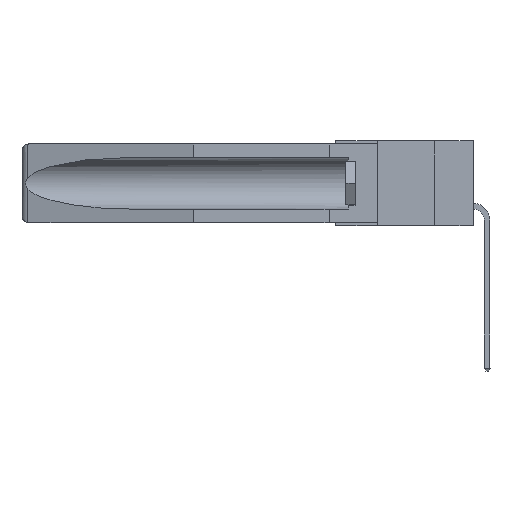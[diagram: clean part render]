
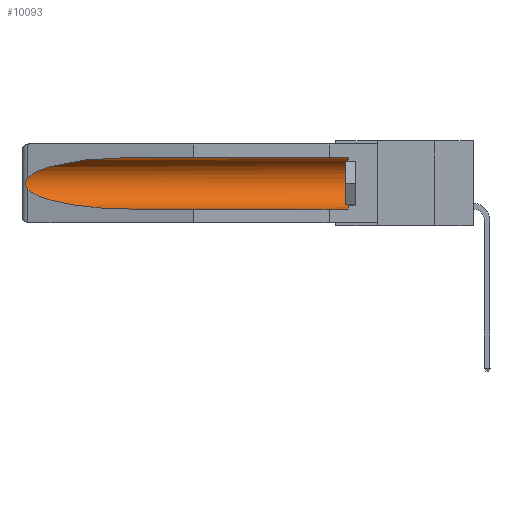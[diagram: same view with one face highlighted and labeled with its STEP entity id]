
A CAD part, left-side view. The second image highlights one B-rep face of the part: STEP entity #10093.
In plain terms, the highlighted cylindrical face has radius 2.857 mm (diameter 5.715 mm), a partial arc.
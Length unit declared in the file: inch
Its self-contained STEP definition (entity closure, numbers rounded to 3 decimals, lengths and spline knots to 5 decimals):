
#797 = VERTEX_POINT ( 'NONE', #23569 ) ;
#885 = AXIS2_PLACEMENT_3D ( 'NONE', #16481, #24147, #20278 ) ;
#1454 = CARTESIAN_POINT ( 'NONE',  ( 0.26654, 1.53092, -0.15636 ) ) ;
#1532 = CARTESIAN_POINT ( 'NONE',  ( 0.2673, 1.53269, -0.17917 ) ) ;
#1546 = DIRECTION ( 'NONE',  ( 0., 1., 0. ) ) ;
#2157 = LINE ( 'NONE', #13804, #13499 ) ;
#2451 = ORIENTED_EDGE ( 'NONE', *, *, #18978, .T. ) ;
#3432 = CARTESIAN_POINT ( 'NONE',  ( 0.2675, 1.53308, -0.17534 ) ) ;
#3751 = CARTESIAN_POINT ( 'NONE',  ( 0.155, -0.30754, -0.1715 ) ) ;
#5003 =( BOUNDED_CURVE ( )  B_SPLINE_CURVE ( 3, ( #21519, #23623, #23539, #6276 ),
 .UNSPECIFIED., .F., .F. ) 
 B_SPLINE_CURVE_WITH_KNOTS ( ( 4, 4 ),
 ( 4.71239, 6.08839 ),
 .UNSPECIFIED. ) 
 CURVE ( )  GEOMETRIC_REPRESENTATION_ITEM ( )  RATIONAL_B_SPLINE_CURVE ( ( 1., 0.848, 0.848, 1. ) ) 
 REPRESENTATION_ITEM ( '' )  );
#5184 = CARTESIAN_POINT ( 'NONE',  ( 0.26597, 1.52961, -0.15275 ) ) ;
#5522 = CARTESIAN_POINT ( 'NONE',  ( 0.155, -0.30754, -0.059 ) ) ;
#5942 = CARTESIAN_POINT ( 'NONE',  ( 0.26537, 1.52718, -0.19328 ) ) ;
#6276 = CARTESIAN_POINT ( 'NONE',  ( 0.26537, 1.52718, -0.14972 ) ) ;
#7214 = VERTEX_POINT ( 'NONE', #7728 ) ;
#7616 =( BOUNDED_CURVE ( )  B_SPLINE_CURVE ( 3, ( #5942, #23096, #16037, #16194 ),
 .UNSPECIFIED., .F., .T. ) 
 B_SPLINE_CURVE_WITH_KNOTS ( ( 4, 4 ),
 ( 0.1948, 1.5708 ),
 .UNSPECIFIED. ) 
 CURVE ( )  GEOMETRIC_REPRESENTATION_ITEM ( )  RATIONAL_B_SPLINE_CURVE ( ( 1., 0.848, 0.848, 1. ) ) 
 REPRESENTATION_ITEM ( '' )  );
#7728 = CARTESIAN_POINT ( 'NONE',  ( 0.155, 1.07973, -0.059 ) ) ;
#9134 = ORIENTED_EDGE ( 'NONE', *, *, #12036, .F. ) ;
#9260 = CARTESIAN_POINT ( 'NONE',  ( 0.155, 1.07973, -0.284 ) ) ;
#9753 = DIRECTION ( 'NONE',  ( 0., 1., 0. ) ) ;
#9761 = VERTEX_POINT ( 'NONE', #20776 ) ;
#10093 = ADVANCED_FACE ( 'NONE', ( #23788 ), #19289, .F. ) ;
#10319 = DIRECTION ( 'NONE',  ( 0., 1., 0. ) ) ;
#10331 = EDGE_LOOP ( 'NONE', ( #11541, #17048, #2451, #9134, #21448, #16360 ) ) ;
#10342 = VERTEX_POINT ( 'NONE', #13432 ) ;
#10353 = CIRCLE ( 'NONE', #885, 0.1125 ) ;
#11541 = ORIENTED_EDGE ( 'NONE', *, *, #14503, .T. ) ;
#11662 = DIRECTION ( 'NONE',  ( 0., 0., 1. ) ) ;
#12036 = EDGE_CURVE ( 'NONE', #14965, #22515, #2157, .T. ) ;
#12930 = CARTESIAN_POINT ( 'NONE',  ( 0.2675, 1.53308, -0.16763 ) ) ;
#12991 = AXIS2_PLACEMENT_3D ( 'NONE', #3751, #9753, #11662 ) ;
#13432 = CARTESIAN_POINT ( 'NONE',  ( 0.155, 0.126, -0.059 ) ) ;
#13499 = VECTOR ( 'NONE', #10319, 39.37008 ) ;
#13804 = CARTESIAN_POINT ( 'NONE',  ( 0.155, -0.30754, -0.284 ) ) ;
#14503 = EDGE_CURVE ( 'NONE', #7214, #797, #5003, .T. ) ;
#14589 = CARTESIAN_POINT ( 'NONE',  ( 0.26597, 1.5296, -0.19026 ) ) ;
#14854 = CARTESIAN_POINT ( 'NONE',  ( 0.26655, 1.53094, -0.18657 ) ) ;
#14965 = VERTEX_POINT ( 'NONE', #22072 ) ;
#15402 = EDGE_CURVE ( 'NONE', #797, #9761, #16033, .T. ) ;
#16033 = B_SPLINE_CURVE_WITH_KNOTS ( 'NONE', 3,
 ( #16861, #5184, #1454, #18606, #12930, #3432, #1532, #14854, #14589, #20589 ),
 .UNSPECIFIED., .F., .F.,
 ( 4, 2, 2, 2, 4 ),
 ( 0., 0.00029, 0.00058, 0.00087, 0.00117 ),
 .UNSPECIFIED. ) ;
#16037 = CARTESIAN_POINT ( 'NONE',  ( 0.21114, 1.30732, -0.284 ) ) ;
#16194 = CARTESIAN_POINT ( 'NONE',  ( 0.155, 1.07973, -0.284 ) ) ;
#16360 = ORIENTED_EDGE ( 'NONE', *, *, #23390, .T. ) ;
#16481 = CARTESIAN_POINT ( 'NONE',  ( 0.155, 0.126, -0.1715 ) ) ;
#16861 = CARTESIAN_POINT ( 'NONE',  ( 0.26537, 1.52718, -0.14972 ) ) ;
#17048 = ORIENTED_EDGE ( 'NONE', *, *, #15402, .T. ) ;
#18606 = CARTESIAN_POINT ( 'NONE',  ( 0.2673, 1.5327, -0.16383 ) ) ;
#18978 = EDGE_CURVE ( 'NONE', #9761, #22515, #7616, .T. ) ;
#19289 = CYLINDRICAL_SURFACE ( 'NONE', #12991, 0.1125 ) ;
#20278 = DIRECTION ( 'NONE',  ( 0., 0., 1. ) ) ;
#20589 = CARTESIAN_POINT ( 'NONE',  ( 0.26537, 1.52718, -0.19328 ) ) ;
#20776 = CARTESIAN_POINT ( 'NONE',  ( 0.26537, 1.52718, -0.19328 ) ) ;
#21448 = ORIENTED_EDGE ( 'NONE', *, *, #22295, .T. ) ;
#21519 = CARTESIAN_POINT ( 'NONE',  ( 0.155, 1.07973, -0.059 ) ) ;
#22072 = CARTESIAN_POINT ( 'NONE',  ( 0.155, 0.126, -0.284 ) ) ;
#22295 = EDGE_CURVE ( 'NONE', #14965, #10342, #10353, .T. ) ;
#22515 = VERTEX_POINT ( 'NONE', #9260 ) ;
#22529 = LINE ( 'NONE', #5522, #22811 ) ;
#22811 = VECTOR ( 'NONE', #1546, 39.37008 ) ;
#23096 = CARTESIAN_POINT ( 'NONE',  ( 0.25451, 1.48313, -0.24835 ) ) ;
#23390 = EDGE_CURVE ( 'NONE', #10342, #7214, #22529, .T. ) ;
#23539 = CARTESIAN_POINT ( 'NONE',  ( 0.25451, 1.48313, -0.09465 ) ) ;
#23569 = CARTESIAN_POINT ( 'NONE',  ( 0.26537, 1.52718, -0.14972 ) ) ;
#23623 = CARTESIAN_POINT ( 'NONE',  ( 0.21114, 1.30732, -0.059 ) ) ;
#23788 = FACE_OUTER_BOUND ( 'NONE', #10331, .T. ) ;
#24147 = DIRECTION ( 'NONE',  ( 0., -1., 0. ) ) ;
